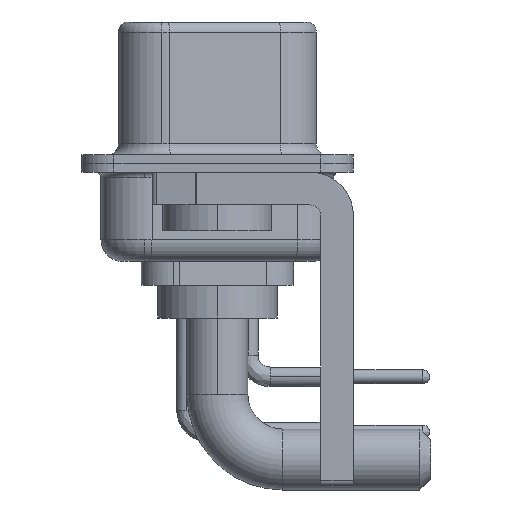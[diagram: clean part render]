
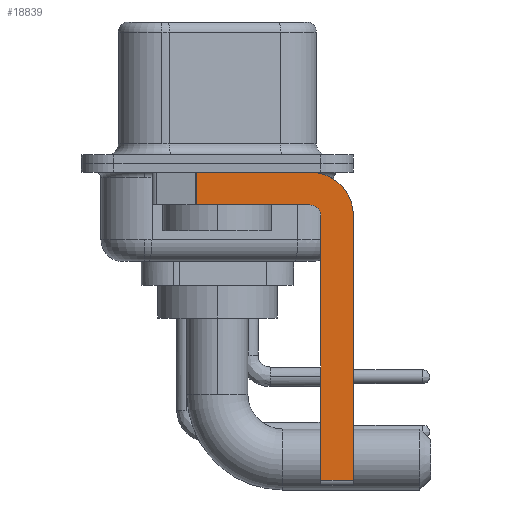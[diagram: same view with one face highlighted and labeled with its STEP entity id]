
A CAD part, left-side view. The second image highlights one B-rep face of the part: STEP entity #18839.
In plain terms, the highlighted planar face has unit normal (-1, 0, 0).
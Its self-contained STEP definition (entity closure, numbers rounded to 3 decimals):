
#177 = VECTOR ( 'NONE', #3436, 1000. ) ;
#195 = VERTEX_POINT ( 'NONE', #12741 ) ;
#431 = EDGE_CURVE ( 'NONE', #1446, #8572, #20258, .T. ) ;
#460 = FACE_OUTER_BOUND ( 'NONE', #2905, .T. ) ;
#822 = ORIENTED_EDGE ( 'NONE', *, *, #16330, .F. ) ;
#1033 = CARTESIAN_POINT ( 'NONE',  ( -2.9, -6.25, -14.55 ) ) ;
#1197 = LINE ( 'NONE', #2547, #5491 ) ;
#1446 = VERTEX_POINT ( 'NONE', #7870 ) ;
#1787 = CARTESIAN_POINT ( 'NONE',  ( -2.9, -4.25, -1.9 ) ) ;
#1900 = DIRECTION ( 'NONE',  ( 0., 1., 0. ) ) ;
#2234 = CARTESIAN_POINT ( 'NONE',  ( -2.9, -4.25, -2.4 ) ) ;
#2429 = CARTESIAN_POINT ( 'NONE',  ( -2.9, 3., -0.4 ) ) ;
#2436 = EDGE_CURVE ( 'NONE', #14901, #21219, #3079, .T. ) ;
#2547 = CARTESIAN_POINT ( 'NONE',  ( -2.9, -4.75, -14.8 ) ) ;
#2738 = ORIENTED_EDGE ( 'NONE', *, *, #7116, .F. ) ;
#2813 = EDGE_CURVE ( 'NONE', #4097, #195, #1197, .T. ) ;
#2905 = EDGE_LOOP ( 'NONE', ( #5427, #20048, #822, #16687, #7817, #14963, #2738, #9649 ) ) ;
#3079 = CIRCLE ( 'NONE', #16161, 2. ) ;
#3436 = DIRECTION ( 'NONE',  ( 0., 0., -1. ) ) ;
#3762 = CARTESIAN_POINT ( 'NONE',  ( -2.9, 0.978, -1.9 ) ) ;
#3779 = VERTEX_POINT ( 'NONE', #1033 ) ;
#3803 = CARTESIAN_POINT ( 'NONE',  ( -2.9, -4.75, -14.55 ) ) ;
#4097 = VERTEX_POINT ( 'NONE', #3803 ) ;
#4245 = AXIS2_PLACEMENT_3D ( 'NONE', #2234, #14071, #5560 ) ;
#4255 = VECTOR ( 'NONE', #15929, 1000. ) ;
#5427 = ORIENTED_EDGE ( 'NONE', *, *, #8766, .F. ) ;
#5491 = VECTOR ( 'NONE', #9709, 1000. ) ;
#5560 = DIRECTION ( 'NONE',  ( 0., 0., -1. ) ) ;
#6033 = VERTEX_POINT ( 'NONE', #19687 ) ;
#6039 = DIRECTION ( 'NONE',  ( -1., 0., 0. ) ) ;
#6124 = DIRECTION ( 'NONE',  ( 1., 0., 0. ) ) ;
#6736 = CIRCLE ( 'NONE', #19792, 0.5 ) ;
#6998 = PLANE ( 'NONE',  #4245 ) ;
#7116 = EDGE_CURVE ( 'NONE', #21219, #3779, #20253, .T. ) ;
#7466 = CARTESIAN_POINT ( 'NONE',  ( -2.9, -4.25, -14.55 ) ) ;
#7817 = ORIENTED_EDGE ( 'NONE', *, *, #2813, .F. ) ;
#7870 = CARTESIAN_POINT ( 'NONE',  ( -2.9, 0.978, -0.4 ) ) ;
#7874 = CARTESIAN_POINT ( 'NONE',  ( -2.9, -4.25, -2.4 ) ) ;
#7899 = DIRECTION ( 'NONE',  ( 0., 0., 1. ) ) ;
#8572 = VERTEX_POINT ( 'NONE', #3762 ) ;
#8766 = EDGE_CURVE ( 'NONE', #1446, #14901, #15710, .T. ) ;
#9649 = ORIENTED_EDGE ( 'NONE', *, *, #2436, .F. ) ;
#9683 = VECTOR ( 'NONE', #16789, 1000. ) ;
#9709 = DIRECTION ( 'NONE',  ( 0., 0., 1. ) ) ;
#10057 = CARTESIAN_POINT ( 'NONE',  ( -2.9, 0.978, -1.9 ) ) ;
#10779 = EDGE_CURVE ( 'NONE', #195, #6033, #6736, .T. ) ;
#11596 = CARTESIAN_POINT ( 'NONE',  ( -2.9, -4.25, -0.4 ) ) ;
#12741 = CARTESIAN_POINT ( 'NONE',  ( -2.9, -4.75, -2.4 ) ) ;
#13639 = EDGE_CURVE ( 'NONE', #4097, #3779, #15878, .T. ) ;
#14071 = DIRECTION ( 'NONE',  ( 1., 0., 0. ) ) ;
#14076 = VECTOR ( 'NONE', #20584, 1000. ) ;
#14901 = VERTEX_POINT ( 'NONE', #11596 ) ;
#14963 = ORIENTED_EDGE ( 'NONE', *, *, #13639, .T. ) ;
#15710 = LINE ( 'NONE', #2429, #4255 ) ;
#15878 = LINE ( 'NONE', #7466, #9683 ) ;
#15929 = DIRECTION ( 'NONE',  ( 0., -1., 0. ) ) ;
#16093 = CARTESIAN_POINT ( 'NONE',  ( -2.9, -4.25, -2.4 ) ) ;
#16161 = AXIS2_PLACEMENT_3D ( 'NONE', #7874, #6124, #17940 ) ;
#16330 = EDGE_CURVE ( 'NONE', #6033, #8572, #20379, .T. ) ;
#16687 = ORIENTED_EDGE ( 'NONE', *, *, #10779, .F. ) ;
#16789 = DIRECTION ( 'NONE',  ( 0., -1., 0. ) ) ;
#17940 = DIRECTION ( 'NONE',  ( 0., 0., -1. ) ) ;
#17989 = VECTOR ( 'NONE', #1900, 1000. ) ;
#18839 = ADVANCED_FACE ( 'NONE', ( #460 ), #6998, .F. ) ;
#19687 = CARTESIAN_POINT ( 'NONE',  ( -2.9, -4.25, -1.9 ) ) ;
#19792 = AXIS2_PLACEMENT_3D ( 'NONE', #16093, #6039, #7899 ) ;
#20048 = ORIENTED_EDGE ( 'NONE', *, *, #431, .T. ) ;
#20084 = CARTESIAN_POINT ( 'NONE',  ( -2.9, -6.25, -2.4 ) ) ;
#20136 = CARTESIAN_POINT ( 'NONE',  ( -2.9, -6.25, -2.4 ) ) ;
#20253 = LINE ( 'NONE', #20136, #14076 ) ;
#20258 = LINE ( 'NONE', #10057, #177 ) ;
#20379 = LINE ( 'NONE', #1787, #17989 ) ;
#20584 = DIRECTION ( 'NONE',  ( 0., 0., -1. ) ) ;
#21219 = VERTEX_POINT ( 'NONE', #20084 ) ;
